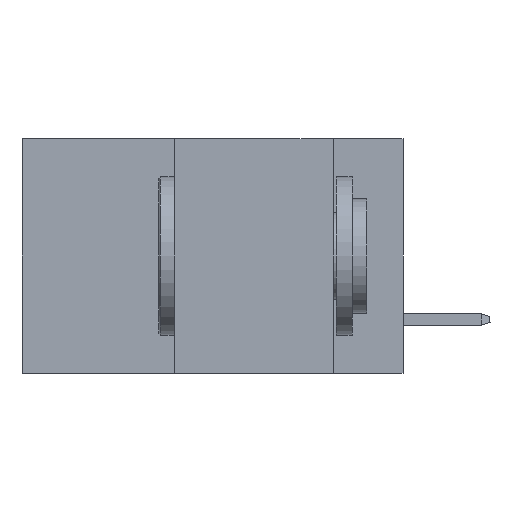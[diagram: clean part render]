
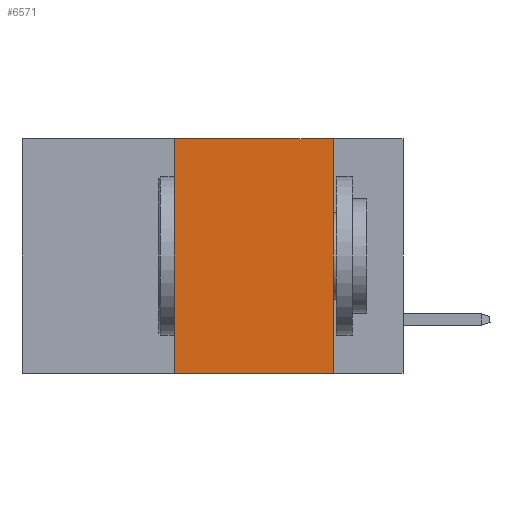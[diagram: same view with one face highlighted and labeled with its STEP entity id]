
A CAD part, left-side view. The second image highlights one B-rep face of the part: STEP entity #6571.
In plain terms, the highlighted planar face has unit normal (-1, 0, 0).
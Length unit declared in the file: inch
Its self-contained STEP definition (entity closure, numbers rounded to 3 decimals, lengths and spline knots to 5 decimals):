
#3286 = EDGE_CURVE ( 'NONE', #9842, #12560, #15168, .T. ) ;
#4139 = CARTESIAN_POINT ( 'NONE',  ( 0., 0.36, -0.37 ) ) ;
#6571 = ADVANCED_FACE ( 'NONE', ( #26136 ), #31646, .F. ) ;
#7062 = CARTESIAN_POINT ( 'NONE',  ( 0., 0.11, 0. ) ) ;
#9109 = CARTESIAN_POINT ( 'NONE',  ( 0., 0.11, -0.37 ) ) ;
#9842 = VERTEX_POINT ( 'NONE', #4139 ) ;
#11575 = EDGE_CURVE ( 'NONE', #9842, #26431, #15979, .T. ) ;
#12560 = VERTEX_POINT ( 'NONE', #9109 ) ;
#12964 = CARTESIAN_POINT ( 'NONE',  ( 0., 0.36, 0. ) ) ;
#14665 = CARTESIAN_POINT ( 'NONE',  ( 0., 0.6, 0. ) ) ;
#15168 = LINE ( 'NONE', #25531, #15481 ) ;
#15481 = VECTOR ( 'NONE', #22844, 39.37008 ) ;
#15979 = LINE ( 'NONE', #12964, #23761 ) ;
#16873 = EDGE_CURVE ( 'NONE', #21569, #12560, #30471, .T. ) ;
#17732 = AXIS2_PLACEMENT_3D ( 'NONE', #31326, #31150, #28649 ) ;
#17749 = DIRECTION ( 'NONE',  ( 0., 0., -1. ) ) ;
#19946 = EDGE_CURVE ( 'NONE', #26431, #21569, #32562, .T. ) ;
#20826 = VECTOR ( 'NONE', #17749, 39.37008 ) ;
#21569 = VERTEX_POINT ( 'NONE', #7062 ) ;
#22844 = DIRECTION ( 'NONE',  ( 0., -1., 0. ) ) ;
#23419 = ORIENTED_EDGE ( 'NONE', *, *, #3286, .T. ) ;
#23761 = VECTOR ( 'NONE', #28352, 39.37008 ) ;
#24634 = ORIENTED_EDGE ( 'NONE', *, *, #11575, .F. ) ;
#24897 = CARTESIAN_POINT ( 'NONE',  ( 0., 0.36, 0. ) ) ;
#25531 = CARTESIAN_POINT ( 'NONE',  ( 0., 0.6, -0.37 ) ) ;
#26136 = FACE_OUTER_BOUND ( 'NONE', #26438, .T. ) ;
#26431 = VERTEX_POINT ( 'NONE', #24897 ) ;
#26438 = EDGE_LOOP ( 'NONE', ( #32997, #30391, #24634, #23419 ) ) ;
#28352 = DIRECTION ( 'NONE',  ( 0., 0., 1. ) ) ;
#28448 = CARTESIAN_POINT ( 'NONE',  ( 0., 0.11, 0. ) ) ;
#28649 = DIRECTION ( 'NONE',  ( 0., 0., -1. ) ) ;
#30062 = VECTOR ( 'NONE', #30223, 39.37008 ) ;
#30223 = DIRECTION ( 'NONE',  ( 0., -1., 0. ) ) ;
#30391 = ORIENTED_EDGE ( 'NONE', *, *, #19946, .F. ) ;
#30471 = LINE ( 'NONE', #28448, #20826 ) ;
#31150 = DIRECTION ( 'NONE',  ( 1., 0., 0. ) ) ;
#31326 = CARTESIAN_POINT ( 'NONE',  ( 0., 0.6, 0. ) ) ;
#31646 = PLANE ( 'NONE',  #17732 ) ;
#32562 = LINE ( 'NONE', #14665, #30062 ) ;
#32997 = ORIENTED_EDGE ( 'NONE', *, *, #16873, .F. ) ;
